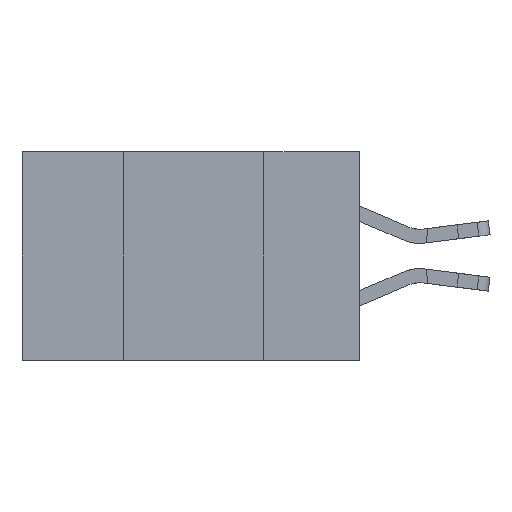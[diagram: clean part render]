
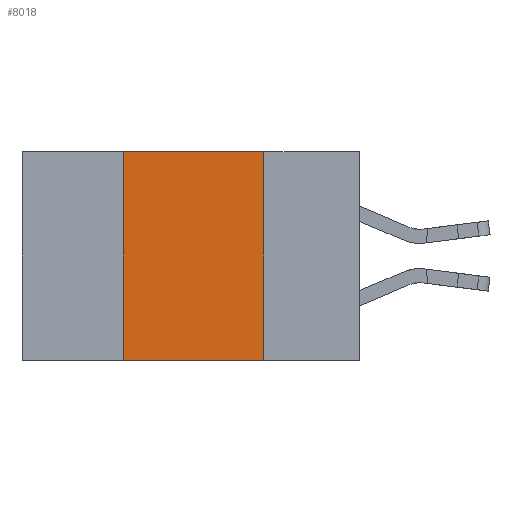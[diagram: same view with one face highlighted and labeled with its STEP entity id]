
A CAD part, left-side view. The second image highlights one B-rep face of the part: STEP entity #8018.
In plain terms, the highlighted planar face has unit normal (-1, 0, 0).
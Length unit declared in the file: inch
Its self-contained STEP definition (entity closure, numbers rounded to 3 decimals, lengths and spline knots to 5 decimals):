
#588 = VERTEX_POINT ( 'NONE', #9277 ) ;
#771 = ORIENTED_EDGE ( 'NONE', *, *, #1717, .F. ) ;
#1175 = LINE ( 'NONE', #17767, #2524 ) ;
#1278 = AXIS2_PLACEMENT_3D ( 'NONE', #17285, #10013, #9634 ) ;
#1532 = ORIENTED_EDGE ( 'NONE', *, *, #9999, .T. ) ;
#1717 = EDGE_CURVE ( 'NONE', #7216, #588, #1175, .T. ) ;
#1730 = CARTESIAN_POINT ( 'NONE',  ( 0., 0.17, 0. ) ) ;
#2524 = VECTOR ( 'NONE', #13262, 39.37008 ) ;
#3046 = DIRECTION ( 'NONE',  ( 0., 0., -1. ) ) ;
#3070 = ORIENTED_EDGE ( 'NONE', *, *, #13943, .F. ) ;
#4344 = VECTOR ( 'NONE', #15611, 39.37008 ) ;
#5096 = VECTOR ( 'NONE', #3046, 39.37008 ) ;
#5159 = EDGE_LOOP ( 'NONE', ( #3070, #12780, #771, #1532 ) ) ;
#6771 = LINE ( 'NONE', #17090, #15598 ) ;
#7216 = VERTEX_POINT ( 'NONE', #11699 ) ;
#7983 = EDGE_CURVE ( 'NONE', #588, #16790, #6771, .T. ) ;
#8018 = ADVANCED_FACE ( 'NONE', ( #17000 ), #8293, .F. ) ;
#8293 = PLANE ( 'NONE',  #1278 ) ;
#8615 = VERTEX_POINT ( 'NONE', #10373 ) ;
#9277 = CARTESIAN_POINT ( 'NONE',  ( 0., 0.42, 0. ) ) ;
#9294 = CARTESIAN_POINT ( 'NONE',  ( 0., 0.17, 0. ) ) ;
#9634 = DIRECTION ( 'NONE',  ( 0., 0., -1. ) ) ;
#9824 = DIRECTION ( 'NONE',  ( 0., -1., 0. ) ) ;
#9999 = EDGE_CURVE ( 'NONE', #7216, #8615, #18312, .T. ) ;
#10013 = DIRECTION ( 'NONE',  ( 1., 0., 0. ) ) ;
#10373 = CARTESIAN_POINT ( 'NONE',  ( 0., 0.17, -0.37 ) ) ;
#11699 = CARTESIAN_POINT ( 'NONE',  ( 0., 0.42, -0.37 ) ) ;
#12458 = CARTESIAN_POINT ( 'NONE',  ( 0., 0.6, -0.37 ) ) ;
#12780 = ORIENTED_EDGE ( 'NONE', *, *, #7983, .F. ) ;
#13262 = DIRECTION ( 'NONE',  ( 0., 0., 1. ) ) ;
#13943 = EDGE_CURVE ( 'NONE', #16790, #8615, #14798, .T. ) ;
#14798 = LINE ( 'NONE', #1730, #5096 ) ;
#15598 = VECTOR ( 'NONE', #9824, 39.37008 ) ;
#15611 = DIRECTION ( 'NONE',  ( 0., -1., 0. ) ) ;
#16790 = VERTEX_POINT ( 'NONE', #9294 ) ;
#17000 = FACE_OUTER_BOUND ( 'NONE', #5159, .T. ) ;
#17090 = CARTESIAN_POINT ( 'NONE',  ( 0., 0.6, 0. ) ) ;
#17285 = CARTESIAN_POINT ( 'NONE',  ( 0., 0.6, 0. ) ) ;
#17767 = CARTESIAN_POINT ( 'NONE',  ( 0., 0.42, 0. ) ) ;
#18312 = LINE ( 'NONE', #12458, #4344 ) ;
